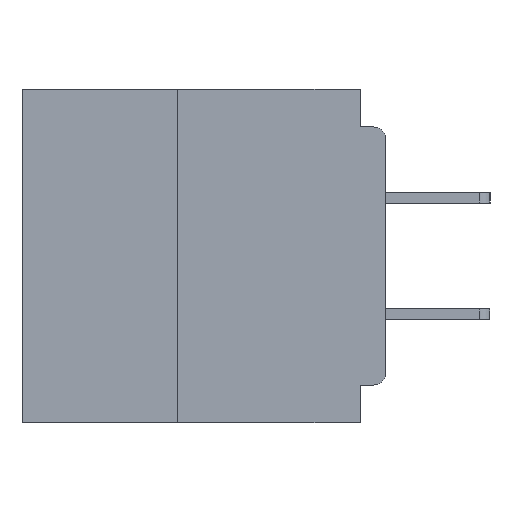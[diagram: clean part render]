
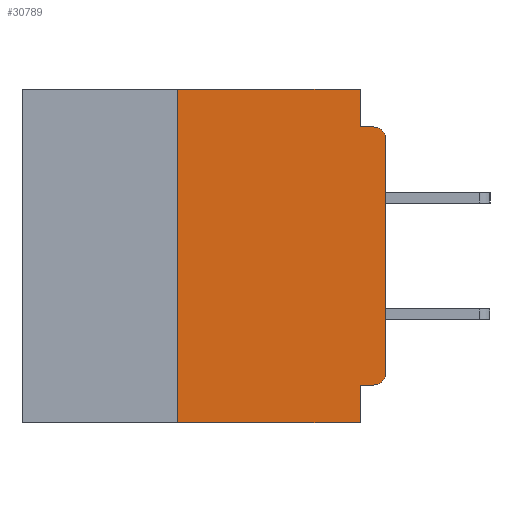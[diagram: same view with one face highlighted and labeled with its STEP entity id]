
A CAD part, left-side view. The second image highlights one B-rep face of the part: STEP entity #30789.
In plain terms, the highlighted planar face has unit normal (-1, 0, 0).
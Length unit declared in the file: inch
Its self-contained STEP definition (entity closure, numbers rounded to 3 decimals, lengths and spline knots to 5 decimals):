
#159 = VERTEX_POINT ( 'NONE', #25150 ) ;
#783 = CARTESIAN_POINT ( 'NONE',  ( 0., 0., -0.34 ) ) ;
#1191 = VERTEX_POINT ( 'NONE', #43330 ) ;
#1237 = CARTESIAN_POINT ( 'NONE',  ( 0., 0.031, 0. ) ) ;
#1268 = DIRECTION ( 'NONE',  ( 0., 0., -1. ) ) ;
#2765 = EDGE_CURVE ( 'NONE', #8384, #3663, #5175, .T. ) ;
#3663 = VERTEX_POINT ( 'NONE', #5832 ) ;
#5175 = LINE ( 'NONE', #31888, #39587 ) ;
#5832 = CARTESIAN_POINT ( 'NONE',  ( 0., 0.25, 0. ) ) ;
#7134 = VECTOR ( 'NONE', #16027, 39.37008 ) ;
#8384 = VERTEX_POINT ( 'NONE', #37963 ) ;
#8666 = CARTESIAN_POINT ( 'NONE',  ( 0., 0.015, -0.06 ) ) ;
#9236 = DIRECTION ( 'NONE',  ( 0., -1., 0. ) ) ;
#9252 = CARTESIAN_POINT ( 'NONE',  ( 0., 0.031, -0.4 ) ) ;
#9324 = EDGE_CURVE ( 'NONE', #3663, #159, #24964, .T. ) ;
#9637 = EDGE_CURVE ( 'NONE', #13892, #15152, #29254, .T. ) ;
#9981 = DIRECTION ( 'NONE',  ( -1., 0., 0. ) ) ;
#10410 = VECTOR ( 'NONE', #33616, 39.37008 ) ;
#10726 = LINE ( 'NONE', #36826, #27979 ) ;
#11387 = EDGE_CURVE ( 'NONE', #15152, #15870, #16376, .T. ) ;
#12137 = DIRECTION ( 'NONE',  ( 0., 0., -1. ) ) ;
#12341 = AXIS2_PLACEMENT_3D ( 'NONE', #30600, #9981, #33990 ) ;
#12726 = EDGE_LOOP ( 'NONE', ( #14016, #16287, #21839, #33384, #41452, #40928, #38171, #30129, #13759, #27983 ) ) ;
#13759 = ORIENTED_EDGE ( 'NONE', *, *, #9637, .F. ) ;
#13892 = VERTEX_POINT ( 'NONE', #18884 ) ;
#14016 = ORIENTED_EDGE ( 'NONE', *, *, #29815, .T. ) ;
#15152 = VERTEX_POINT ( 'NONE', #39415 ) ;
#15451 = DIRECTION ( 'NONE',  ( 0., -1., 0. ) ) ;
#15870 = VERTEX_POINT ( 'NONE', #9252 ) ;
#16027 = DIRECTION ( 'NONE',  ( 0., 0., -1. ) ) ;
#16287 = ORIENTED_EDGE ( 'NONE', *, *, #34299, .T. ) ;
#16295 = DIRECTION ( 'NONE',  ( 0., -1., 0. ) ) ;
#16376 = LINE ( 'NONE', #26281, #7134 ) ;
#17327 = FACE_OUTER_BOUND ( 'NONE', #12726, .T. ) ;
#17775 = LINE ( 'NONE', #1237, #25876 ) ;
#18518 = PLANE ( 'NONE',  #39698 ) ;
#18884 = CARTESIAN_POINT ( 'NONE',  ( 0., 0.015, -0.355 ) ) ;
#21117 = VECTOR ( 'NONE', #40969, 39.37008 ) ;
#21839 = ORIENTED_EDGE ( 'NONE', *, *, #30367, .F. ) ;
#21983 = DIRECTION ( 'NONE',  ( 1., 0., 0. ) ) ;
#22061 = CIRCLE ( 'NONE', #12341, 0.015 ) ;
#22929 = LINE ( 'NONE', #26433, #26564 ) ;
#23252 = EDGE_CURVE ( 'NONE', #159, #1191, #17775, .T. ) ;
#24721 = CARTESIAN_POINT ( 'NONE',  ( 0., 0., -0.06 ) ) ;
#24961 = AXIS2_PLACEMENT_3D ( 'NONE', #8666, #32726, #12137 ) ;
#24964 = LINE ( 'NONE', #39400, #41951 ) ;
#25131 = DIRECTION ( 'NONE',  ( 0., 0., 1. ) ) ;
#25150 = CARTESIAN_POINT ( 'NONE',  ( 0., 0.031, 0. ) ) ;
#25876 = VECTOR ( 'NONE', #28916, 39.37008 ) ;
#26281 = CARTESIAN_POINT ( 'NONE',  ( 0., 0.031, -0.4 ) ) ;
#26433 = CARTESIAN_POINT ( 'NONE',  ( 0., 0., -0.045 ) ) ;
#26564 = VECTOR ( 'NONE', #9236, 39.37008 ) ;
#27719 = VERTEX_POINT ( 'NONE', #783 ) ;
#27979 = VECTOR ( 'NONE', #16295, 39.37008 ) ;
#27983 = ORIENTED_EDGE ( 'NONE', *, *, #42136, .T. ) ;
#28801 = CARTESIAN_POINT ( 'NONE',  ( 0., 0.437, 0. ) ) ;
#28916 = DIRECTION ( 'NONE',  ( 0., 0., -1. ) ) ;
#29254 = LINE ( 'NONE', #30780, #21117 ) ;
#29815 = EDGE_CURVE ( 'NONE', #27719, #31254, #38848, .T. ) ;
#30129 = ORIENTED_EDGE ( 'NONE', *, *, #11387, .F. ) ;
#30367 = EDGE_CURVE ( 'NONE', #1191, #36783, #22929, .T. ) ;
#30600 = CARTESIAN_POINT ( 'NONE',  ( 0., 0.015, -0.34 ) ) ;
#30780 = CARTESIAN_POINT ( 'NONE',  ( 0., 0., -0.355 ) ) ;
#30789 = ADVANCED_FACE ( 'NONE', ( #17327 ), #18518, .F. ) ;
#31254 = VERTEX_POINT ( 'NONE', #24721 ) ;
#31888 = CARTESIAN_POINT ( 'NONE',  ( 0., 0.25, -0.4 ) ) ;
#32726 = DIRECTION ( 'NONE',  ( -1., 0., 0. ) ) ;
#32907 = EDGE_CURVE ( 'NONE', #8384, #15870, #10726, .T. ) ;
#33384 = ORIENTED_EDGE ( 'NONE', *, *, #23252, .F. ) ;
#33616 = DIRECTION ( 'NONE',  ( 0., 0., 1. ) ) ;
#33990 = DIRECTION ( 'NONE',  ( 0., 0., -1. ) ) ;
#34299 = EDGE_CURVE ( 'NONE', #31254, #36783, #42665, .T. ) ;
#36783 = VERTEX_POINT ( 'NONE', #42843 ) ;
#36826 = CARTESIAN_POINT ( 'NONE',  ( 0., 0.437, -0.4 ) ) ;
#37963 = CARTESIAN_POINT ( 'NONE',  ( 0., 0.25, -0.4 ) ) ;
#38171 = ORIENTED_EDGE ( 'NONE', *, *, #32907, .T. ) ;
#38848 = LINE ( 'NONE', #40414, #10410 ) ;
#39400 = CARTESIAN_POINT ( 'NONE',  ( 0., 0.437, 0. ) ) ;
#39415 = CARTESIAN_POINT ( 'NONE',  ( 0., 0.031, -0.355 ) ) ;
#39587 = VECTOR ( 'NONE', #25131, 39.37008 ) ;
#39698 = AXIS2_PLACEMENT_3D ( 'NONE', #28801, #21983, #1268 ) ;
#40414 = CARTESIAN_POINT ( 'NONE',  ( 0., 0., 0. ) ) ;
#40928 = ORIENTED_EDGE ( 'NONE', *, *, #2765, .F. ) ;
#40969 = DIRECTION ( 'NONE',  ( 0., 1., 0. ) ) ;
#41452 = ORIENTED_EDGE ( 'NONE', *, *, #9324, .F. ) ;
#41951 = VECTOR ( 'NONE', #15451, 39.37008 ) ;
#42136 = EDGE_CURVE ( 'NONE', #13892, #27719, #22061, .T. ) ;
#42665 = CIRCLE ( 'NONE', #24961, 0.015 ) ;
#42843 = CARTESIAN_POINT ( 'NONE',  ( 0., 0.015, -0.045 ) ) ;
#43330 = CARTESIAN_POINT ( 'NONE',  ( 0., 0.031, -0.045 ) ) ;
